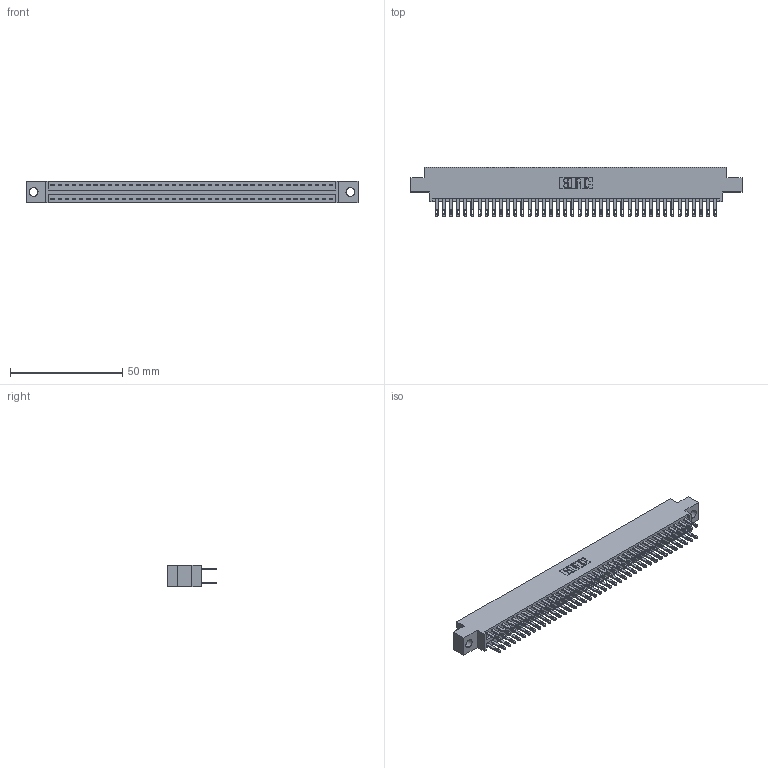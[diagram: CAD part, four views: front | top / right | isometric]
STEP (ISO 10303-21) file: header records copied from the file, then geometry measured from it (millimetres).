
FILE_DESCRIPTION (( 'STEP AP203' ), '1' );
FILE_NAME ('346-080-500-804.STEP', '2018-08-29T06:54:58', ( '' ), ( '' ), 'SwSTEP 2.0', 'SolidWorks 2016', '' );
FILE_SCHEMA (( 'CONFIG_CONTROL_DESIGN' ));
Length unit declared in the file: inch
Products named in the file (3): 346-080-500-804; 346 Part_0.170 Offset - 0.156 Dia-TH; 345-292-001_345-293-100
Assembly tree (81 placements, depth 2):
  346-080-500-804
    346 Part_0.170 Offset - 0.156 Dia-TH
    345-292-001_345-293-100  x80
Bounding box: 147.57 x 21.84 x 9.4 mm (x, y, z)
Volume: 14376.8 mm3; surface area: 20560.7 mm2
Topology: 81 solids, 81 shells, 3966 faces, 12101 edges, 8066 vertices
Faces by surface type: plane 2400, cylinder 1566
Entity records: 26439 total; most frequent: CARTESIAN_POINT 4360, ORIENTED_EDGE 4294, DIRECTION 3895, EDGE_CURVE 2147, VECTOR 1851, LINE 1851, VERTEX_POINT 1430, AXIS2_PLACEMENT_3D 1022
